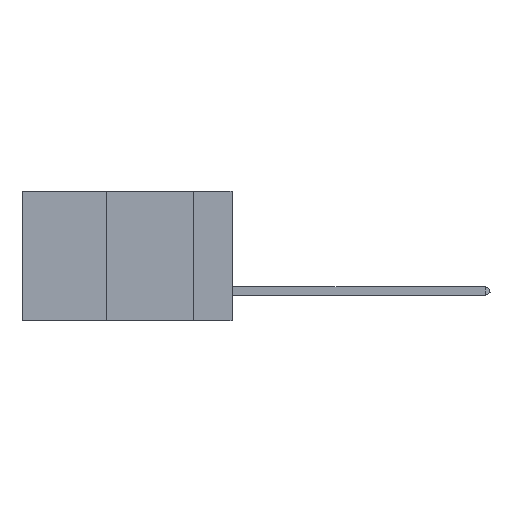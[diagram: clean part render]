
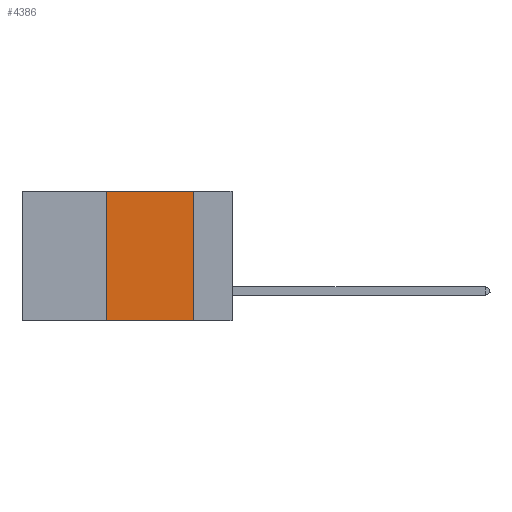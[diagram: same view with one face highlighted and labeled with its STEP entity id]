
A CAD part, left-side view. The second image highlights one B-rep face of the part: STEP entity #4386.
In plain terms, the highlighted planar face has unit normal (-1, 0, 0).
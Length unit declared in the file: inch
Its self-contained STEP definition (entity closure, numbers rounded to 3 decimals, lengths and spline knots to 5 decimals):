
#3449 = CARTESIAN_POINT ( 'NONE',  ( 0., 0.11, 0. ) ) ;
#4386 = ADVANCED_FACE ( 'NONE', ( #7900 ), #47045, .F. ) ;
#5348 = VECTOR ( 'NONE', #32505, 39.37008 ) ;
#5949 = CARTESIAN_POINT ( 'NONE',  ( 0., 0.36, 0. ) ) ;
#7900 = FACE_OUTER_BOUND ( 'NONE', #30941, .T. ) ;
#10602 = LINE ( 'NONE', #15467, #22115 ) ;
#14670 = VERTEX_POINT ( 'NONE', #5949 ) ;
#15467 = CARTESIAN_POINT ( 'NONE',  ( 0., 0.6, -0.37 ) ) ;
#18481 = VERTEX_POINT ( 'NONE', #38194 ) ;
#19249 = EDGE_CURVE ( 'NONE', #24870, #42561, #25423, .T. ) ;
#19556 = LINE ( 'NONE', #42981, #23000 ) ;
#21188 = EDGE_CURVE ( 'NONE', #14670, #24870, #41563, .T. ) ;
#22115 = VECTOR ( 'NONE', #37761, 39.37008 ) ;
#23000 = VECTOR ( 'NONE', #28197, 39.37008 ) ;
#24870 = VERTEX_POINT ( 'NONE', #3449 ) ;
#25423 = LINE ( 'NONE', #43257, #36876 ) ;
#25483 = ORIENTED_EDGE ( 'NONE', *, *, #19249, .F. ) ;
#25761 = ORIENTED_EDGE ( 'NONE', *, *, #43918, .F. ) ;
#26267 = ORIENTED_EDGE ( 'NONE', *, *, #21188, .F. ) ;
#28197 = DIRECTION ( 'NONE',  ( 0., 0., 1. ) ) ;
#29046 = DIRECTION ( 'NONE',  ( 1., 0., 0. ) ) ;
#29196 = CARTESIAN_POINT ( 'NONE',  ( 0., 0.6, 0. ) ) ;
#30941 = EDGE_LOOP ( 'NONE', ( #25483, #26267, #25761, #35264 ) ) ;
#32346 = CARTESIAN_POINT ( 'NONE',  ( 0., 0.6, 0. ) ) ;
#32505 = DIRECTION ( 'NONE',  ( 0., -1., 0. ) ) ;
#34604 = AXIS2_PLACEMENT_3D ( 'NONE', #29196, #29046, #43648 ) ;
#35264 = ORIENTED_EDGE ( 'NONE', *, *, #37000, .T. ) ;
#35684 = DIRECTION ( 'NONE',  ( 0., 0., -1. ) ) ;
#36876 = VECTOR ( 'NONE', #35684, 39.37008 ) ;
#37000 = EDGE_CURVE ( 'NONE', #18481, #42561, #10602, .T. ) ;
#37761 = DIRECTION ( 'NONE',  ( 0., -1., 0. ) ) ;
#37774 = CARTESIAN_POINT ( 'NONE',  ( 0., 0.11, -0.37 ) ) ;
#38194 = CARTESIAN_POINT ( 'NONE',  ( 0., 0.36, -0.37 ) ) ;
#41563 = LINE ( 'NONE', #32346, #5348 ) ;
#42561 = VERTEX_POINT ( 'NONE', #37774 ) ;
#42981 = CARTESIAN_POINT ( 'NONE',  ( 0., 0.36, 0. ) ) ;
#43257 = CARTESIAN_POINT ( 'NONE',  ( 0., 0.11, 0. ) ) ;
#43648 = DIRECTION ( 'NONE',  ( 0., 0., -1. ) ) ;
#43918 = EDGE_CURVE ( 'NONE', #18481, #14670, #19556, .T. ) ;
#47045 = PLANE ( 'NONE',  #34604 ) ;
